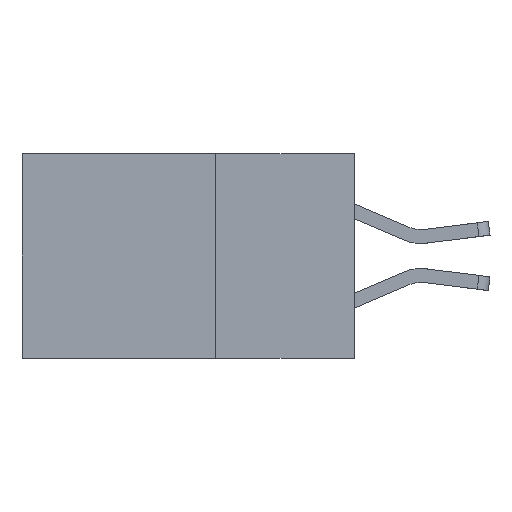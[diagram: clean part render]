
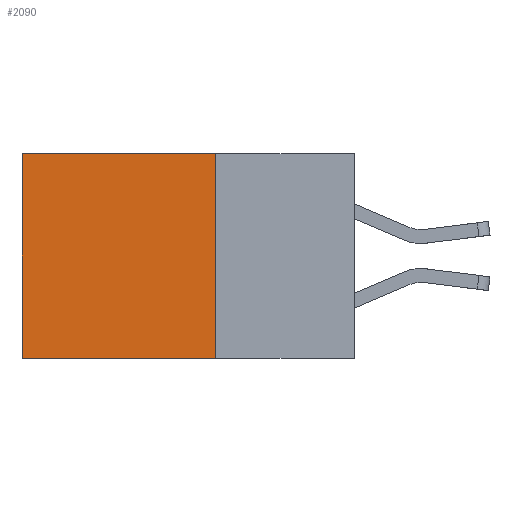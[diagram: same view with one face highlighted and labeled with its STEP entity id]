
A CAD part, left-side view. The second image highlights one B-rep face of the part: STEP entity #2090.
In plain terms, the highlighted planar face has unit normal (-1, 0, 0).
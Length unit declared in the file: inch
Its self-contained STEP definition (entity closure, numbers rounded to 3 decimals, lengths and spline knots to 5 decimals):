
#183 = DIRECTION ( 'NONE',  ( 0., 1., 0. ) ) ;
#1113 = VECTOR ( 'NONE', #8129, 39.37008 ) ;
#1441 = ORIENTED_EDGE ( 'NONE', *, *, #7348, .F. ) ;
#1508 = CARTESIAN_POINT ( 'NONE',  ( 0.298, 0.25, 0. ) ) ;
#1629 = CARTESIAN_POINT ( 'NONE',  ( 0.298, 0.25, 0. ) ) ;
#2064 = VECTOR ( 'NONE', #183, 39.37008 ) ;
#2090 = ADVANCED_FACE ( 'NONE', ( #7914 ), #3368, .F. ) ;
#2176 = EDGE_CURVE ( 'NONE', #9294, #2193, #8226, .T. ) ;
#2193 = VERTEX_POINT ( 'NONE', #4681 ) ;
#2565 = VECTOR ( 'NONE', #6352, 39.37008 ) ;
#2824 = VECTOR ( 'NONE', #4281, 39.37008 ) ;
#3075 = LINE ( 'NONE', #3516, #2824 ) ;
#3368 = PLANE ( 'NONE',  #6541 ) ;
#3428 = ORIENTED_EDGE ( 'NONE', *, *, #8407, .T. ) ;
#3516 = CARTESIAN_POINT ( 'NONE',  ( 0.298, 0.25, 0. ) ) ;
#3637 = CARTESIAN_POINT ( 'NONE',  ( 0.298, 0.6, 0. ) ) ;
#4221 = LINE ( 'NONE', #1629, #2064 ) ;
#4281 = DIRECTION ( 'NONE',  ( 0., 0., -1. ) ) ;
#4681 = CARTESIAN_POINT ( 'NONE',  ( 0.298, 0.6, -0.37 ) ) ;
#4703 = CARTESIAN_POINT ( 'NONE',  ( 0.298, 0.25, -0.37 ) ) ;
#4880 = DIRECTION ( 'NONE',  ( 1., 0., 0. ) ) ;
#5258 = CARTESIAN_POINT ( 'NONE',  ( 0.298, 0.25, 0. ) ) ;
#5288 = CARTESIAN_POINT ( 'NONE',  ( 0.298, 0.6, 0. ) ) ;
#5582 = EDGE_CURVE ( 'NONE', #8383, #8199, #4221, .T. ) ;
#6205 = EDGE_LOOP ( 'NONE', ( #3428, #7292, #1441, #9402 ) ) ;
#6352 = DIRECTION ( 'NONE',  ( 0., 1., 0. ) ) ;
#6541 = AXIS2_PLACEMENT_3D ( 'NONE', #1508, #4880, #8048 ) ;
#7224 = LINE ( 'NONE', #5288, #1113 ) ;
#7292 = ORIENTED_EDGE ( 'NONE', *, *, #2176, .F. ) ;
#7348 = EDGE_CURVE ( 'NONE', #8383, #9294, #3075, .T. ) ;
#7914 = FACE_OUTER_BOUND ( 'NONE', #6205, .T. ) ;
#8048 = DIRECTION ( 'NONE',  ( 0., 0., -1. ) ) ;
#8129 = DIRECTION ( 'NONE',  ( 0., 0., -1. ) ) ;
#8199 = VERTEX_POINT ( 'NONE', #3637 ) ;
#8226 = LINE ( 'NONE', #4703, #2565 ) ;
#8383 = VERTEX_POINT ( 'NONE', #5258 ) ;
#8407 = EDGE_CURVE ( 'NONE', #8199, #2193, #7224, .T. ) ;
#9089 = CARTESIAN_POINT ( 'NONE',  ( 0.298, 0.25, -0.37 ) ) ;
#9294 = VERTEX_POINT ( 'NONE', #9089 ) ;
#9402 = ORIENTED_EDGE ( 'NONE', *, *, #5582, .T. ) ;
